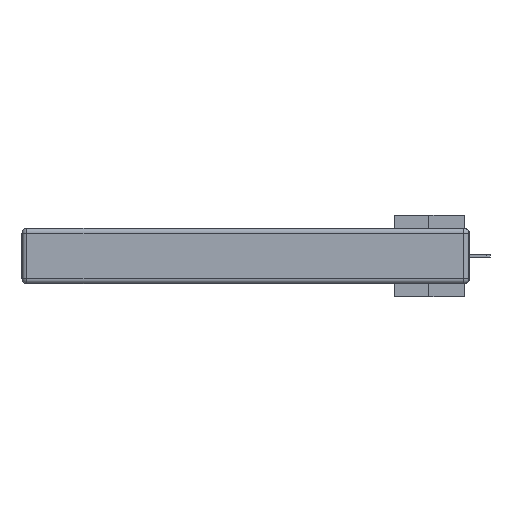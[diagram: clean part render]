
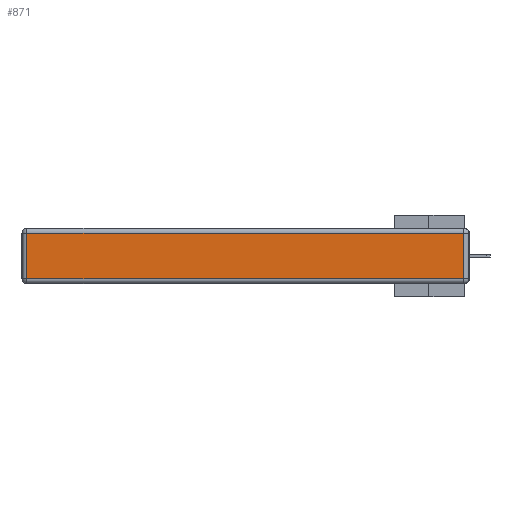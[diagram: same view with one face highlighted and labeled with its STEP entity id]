
A CAD part, left-side view. The second image highlights one B-rep face of the part: STEP entity #871.
In plain terms, the highlighted planar face has unit normal (-1, 0, 0).
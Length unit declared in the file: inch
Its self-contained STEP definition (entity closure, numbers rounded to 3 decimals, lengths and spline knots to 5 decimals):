
#450 = CARTESIAN_POINT ( 'NONE',  ( 0., 0., -0.313 ) ) ;
#871 = ADVANCED_FACE ( 'NONE', ( #17920 ), #17353, .T. ) ;
#1306 = LINE ( 'NONE', #16203, #31739 ) ;
#1877 = VERTEX_POINT ( 'NONE', #21866 ) ;
#1956 = ORIENTED_EDGE ( 'NONE', *, *, #12505, .T. ) ;
#2518 = EDGE_CURVE ( 'NONE', #1877, #19636, #1306, .T. ) ;
#2913 = CARTESIAN_POINT ( 'NONE',  ( 0., 2.72, -0.03 ) ) ;
#3134 = CARTESIAN_POINT ( 'NONE',  ( 0., 0.03, -0.313 ) ) ;
#3305 = EDGE_CURVE ( 'NONE', #6200, #31234, #20722, .T. ) ;
#4184 = DIRECTION ( 'NONE',  ( 0., 0., -1. ) ) ;
#4989 = DIRECTION ( 'NONE',  ( 0., 0., 1. ) ) ;
#5083 = VECTOR ( 'NONE', #21098, 39.37008 ) ;
#5693 = DIRECTION ( 'NONE',  ( 0., 0., 1. ) ) ;
#6200 = VERTEX_POINT ( 'NONE', #12772 ) ;
#6255 = AXIS2_PLACEMENT_3D ( 'NONE', #29650, #37888, #5693 ) ;
#8683 = EDGE_LOOP ( 'NONE', ( #37064, #32721, #8860, #1956 ) ) ;
#8860 = ORIENTED_EDGE ( 'NONE', *, *, #2518, .T. ) ;
#11678 = CARTESIAN_POINT ( 'NONE',  ( 0., 2.72, -0.343 ) ) ;
#12505 = EDGE_CURVE ( 'NONE', #19636, #6200, #27764, .T. ) ;
#12772 = CARTESIAN_POINT ( 'NONE',  ( 0., 2.72, -0.313 ) ) ;
#16203 = CARTESIAN_POINT ( 'NONE',  ( 0., 2.75, -0.03 ) ) ;
#16567 = VECTOR ( 'NONE', #4989, 39.37008 ) ;
#17353 = PLANE ( 'NONE',  #6255 ) ;
#17920 = FACE_OUTER_BOUND ( 'NONE', #8683, .T. ) ;
#18508 = VECTOR ( 'NONE', #4184, 39.37008 ) ;
#19636 = VERTEX_POINT ( 'NONE', #2913 ) ;
#20722 = LINE ( 'NONE', #450, #5083 ) ;
#21098 = DIRECTION ( 'NONE',  ( 0., -1., 0. ) ) ;
#21585 = DIRECTION ( 'NONE',  ( 0., 1., 0. ) ) ;
#21866 = CARTESIAN_POINT ( 'NONE',  ( 0., 0.03, -0.03 ) ) ;
#22305 = EDGE_CURVE ( 'NONE', #31234, #1877, #31240, .T. ) ;
#27764 = LINE ( 'NONE', #11678, #18508 ) ;
#29650 = CARTESIAN_POINT ( 'NONE',  ( 0., 0., -0.343 ) ) ;
#31234 = VERTEX_POINT ( 'NONE', #3134 ) ;
#31240 = LINE ( 'NONE', #31603, #16567 ) ;
#31603 = CARTESIAN_POINT ( 'NONE',  ( 0., 0.03, -0.343 ) ) ;
#31739 = VECTOR ( 'NONE', #21585, 39.37008 ) ;
#32721 = ORIENTED_EDGE ( 'NONE', *, *, #22305, .T. ) ;
#37064 = ORIENTED_EDGE ( 'NONE', *, *, #3305, .T. ) ;
#37888 = DIRECTION ( 'NONE',  ( -1., 0., 0. ) ) ;
